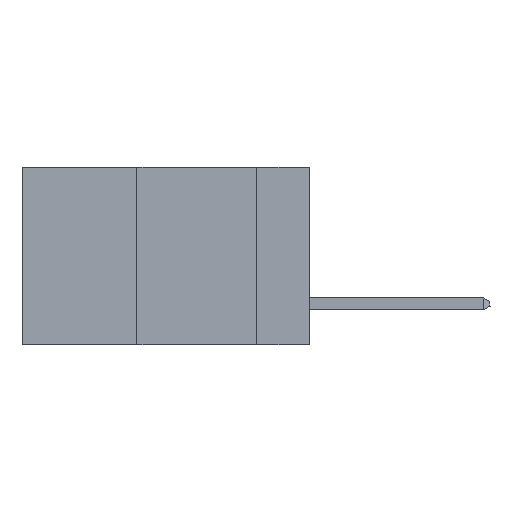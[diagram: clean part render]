
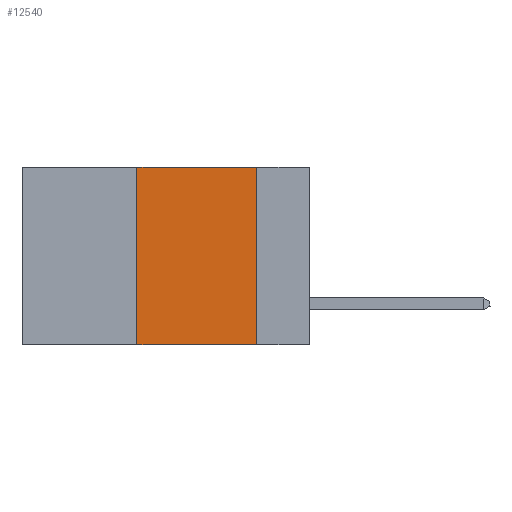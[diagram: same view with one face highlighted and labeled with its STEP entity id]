
A CAD part, left-side view. The second image highlights one B-rep face of the part: STEP entity #12540.
In plain terms, the highlighted planar face has unit normal (-1, 0, 0).
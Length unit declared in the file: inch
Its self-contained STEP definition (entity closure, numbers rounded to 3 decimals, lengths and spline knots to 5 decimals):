
#85 = ORIENTED_EDGE ( 'NONE', *, *, #2020, .F. ) ;
#563 = DIRECTION ( 'NONE',  ( 0., -1., 0. ) ) ;
#767 = CARTESIAN_POINT ( 'NONE',  ( 0., 0.36, 0. ) ) ;
#1243 = CARTESIAN_POINT ( 'NONE',  ( 0., 0.36, 0. ) ) ;
#1262 = CARTESIAN_POINT ( 'NONE',  ( 0., 0.6, 0. ) ) ;
#1637 = LINE ( 'NONE', #1262, #1956 ) ;
#1755 = FACE_OUTER_BOUND ( 'NONE', #10106, .T. ) ;
#1956 = VECTOR ( 'NONE', #13079, 39.37008 ) ;
#2020 = EDGE_CURVE ( 'NONE', #10815, #4592, #13322, .T. ) ;
#3157 = CARTESIAN_POINT ( 'NONE',  ( 0., 0.11, 0. ) ) ;
#3303 = EDGE_CURVE ( 'NONE', #5348, #4592, #13515, .T. ) ;
#3407 = DIRECTION ( 'NONE',  ( 0., 0., 1. ) ) ;
#4275 = VERTEX_POINT ( 'NONE', #767 ) ;
#4566 = ORIENTED_EDGE ( 'NONE', *, *, #10568, .F. ) ;
#4592 = VERTEX_POINT ( 'NONE', #7896 ) ;
#5263 = VECTOR ( 'NONE', #3407, 39.37008 ) ;
#5348 = VERTEX_POINT ( 'NONE', #8405 ) ;
#5382 = ORIENTED_EDGE ( 'NONE', *, *, #9532, .F. ) ;
#6085 = AXIS2_PLACEMENT_3D ( 'NONE', #13260, #7893, #7940 ) ;
#6142 = CARTESIAN_POINT ( 'NONE',  ( 0., 0.11, 0. ) ) ;
#7012 = VECTOR ( 'NONE', #13690, 39.37008 ) ;
#7893 = DIRECTION ( 'NONE',  ( 1., 0., 0. ) ) ;
#7896 = CARTESIAN_POINT ( 'NONE',  ( 0., 0.11, -0.37 ) ) ;
#7940 = DIRECTION ( 'NONE',  ( 0., 0., -1. ) ) ;
#8405 = CARTESIAN_POINT ( 'NONE',  ( 0., 0.36, -0.37 ) ) ;
#8467 = VECTOR ( 'NONE', #563, 39.37008 ) ;
#8907 = PLANE ( 'NONE',  #6085 ) ;
#9532 = EDGE_CURVE ( 'NONE', #5348, #4275, #13733, .T. ) ;
#10106 = EDGE_LOOP ( 'NONE', ( #85, #4566, #5382, #12549 ) ) ;
#10232 = CARTESIAN_POINT ( 'NONE',  ( 0., 0.6, -0.37 ) ) ;
#10568 = EDGE_CURVE ( 'NONE', #4275, #10815, #1637, .T. ) ;
#10815 = VERTEX_POINT ( 'NONE', #6142 ) ;
#12540 = ADVANCED_FACE ( 'NONE', ( #1755 ), #8907, .F. ) ;
#12549 = ORIENTED_EDGE ( 'NONE', *, *, #3303, .T. ) ;
#13079 = DIRECTION ( 'NONE',  ( 0., -1., 0. ) ) ;
#13260 = CARTESIAN_POINT ( 'NONE',  ( 0., 0.6, 0. ) ) ;
#13322 = LINE ( 'NONE', #3157, #7012 ) ;
#13515 = LINE ( 'NONE', #10232, #8467 ) ;
#13690 = DIRECTION ( 'NONE',  ( 0., 0., -1. ) ) ;
#13733 = LINE ( 'NONE', #1243, #5263 ) ;
